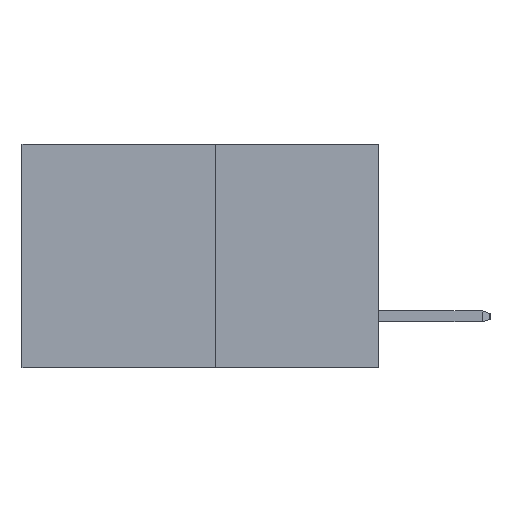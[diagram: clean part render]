
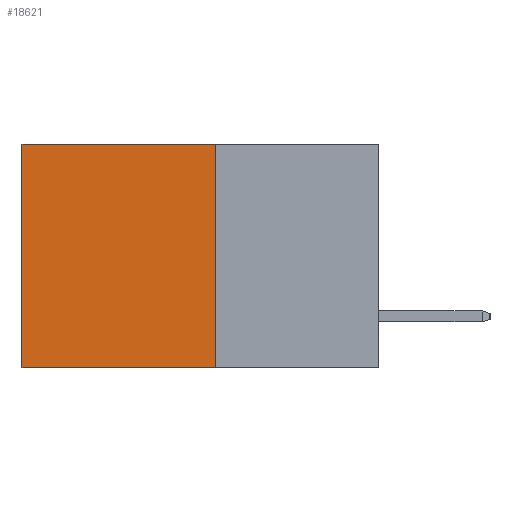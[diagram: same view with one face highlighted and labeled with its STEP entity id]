
A CAD part, left-side view. The second image highlights one B-rep face of the part: STEP entity #18621.
In plain terms, the highlighted planar face has unit normal (-1, 0, 0).
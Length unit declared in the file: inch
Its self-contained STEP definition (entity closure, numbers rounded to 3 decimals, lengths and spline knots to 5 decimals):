
#834 = VERTEX_POINT ( 'NONE', #16503 ) ;
#1132 = EDGE_CURVE ( 'NONE', #6788, #2710, #21112, .T. ) ;
#1731 = CARTESIAN_POINT ( 'NONE',  ( 0.277, 0.59, -0.37 ) ) ;
#1833 = CARTESIAN_POINT ( 'NONE',  ( 0.277, 0.59, -0.37 ) ) ;
#2314 = EDGE_CURVE ( 'NONE', #18376, #6788, #8640, .T. ) ;
#2361 = VECTOR ( 'NONE', #18084, 39.37008 ) ;
#2472 = VECTOR ( 'NONE', #8204, 39.37008 ) ;
#2710 = VERTEX_POINT ( 'NONE', #1833 ) ;
#3567 = VECTOR ( 'NONE', #4571, 39.37008 ) ;
#4149 = EDGE_CURVE ( 'NONE', #18376, #834, #11576, .T. ) ;
#4571 = DIRECTION ( 'NONE',  ( 0., 1., 0. ) ) ;
#6788 = VERTEX_POINT ( 'NONE', #21960 ) ;
#7068 = CARTESIAN_POINT ( 'NONE',  ( 0.277, 0.27, -0.37 ) ) ;
#7299 = EDGE_CURVE ( 'NONE', #834, #2710, #15792, .T. ) ;
#7732 = ORIENTED_EDGE ( 'NONE', *, *, #1132, .T. ) ;
#8204 = DIRECTION ( 'NONE',  ( 0., 1., 0. ) ) ;
#8294 = CARTESIAN_POINT ( 'NONE',  ( 0.277, 0.27, -0.37 ) ) ;
#8640 = LINE ( 'NONE', #11013, #3567 ) ;
#9140 = DIRECTION ( 'NONE',  ( 1., 0., 0. ) ) ;
#11013 = CARTESIAN_POINT ( 'NONE',  ( 0.277, 0.27, 0. ) ) ;
#11576 = LINE ( 'NONE', #7068, #2361 ) ;
#13588 = ORIENTED_EDGE ( 'NONE', *, *, #2314, .T. ) ;
#13690 = ORIENTED_EDGE ( 'NONE', *, *, #4149, .F. ) ;
#14389 = PLANE ( 'NONE',  #19515 ) ;
#15497 = ORIENTED_EDGE ( 'NONE', *, *, #7299, .F. ) ;
#15540 = CARTESIAN_POINT ( 'NONE',  ( 0.277, 0.27, 0. ) ) ;
#15641 = EDGE_LOOP ( 'NONE', ( #7732, #15497, #13690, #13588 ) ) ;
#15663 = FACE_OUTER_BOUND ( 'NONE', #15641, .T. ) ;
#15792 = LINE ( 'NONE', #8294, #2472 ) ;
#15941 = DIRECTION ( 'NONE',  ( 0., 0., -1. ) ) ;
#16503 = CARTESIAN_POINT ( 'NONE',  ( 0.277, 0.27, -0.37 ) ) ;
#17160 = VECTOR ( 'NONE', #15941, 39.37008 ) ;
#18084 = DIRECTION ( 'NONE',  ( 0., 0., -1. ) ) ;
#18376 = VERTEX_POINT ( 'NONE', #15540 ) ;
#18621 = ADVANCED_FACE ( 'NONE', ( #15663 ), #14389, .F. ) ;
#19515 = AXIS2_PLACEMENT_3D ( 'NONE', #19537, #9140, #21214 ) ;
#19537 = CARTESIAN_POINT ( 'NONE',  ( 0.277, 0.27, -0.37 ) ) ;
#21112 = LINE ( 'NONE', #1731, #17160 ) ;
#21214 = DIRECTION ( 'NONE',  ( 0., 0., -1. ) ) ;
#21960 = CARTESIAN_POINT ( 'NONE',  ( 0.277, 0.59, 0. ) ) ;
